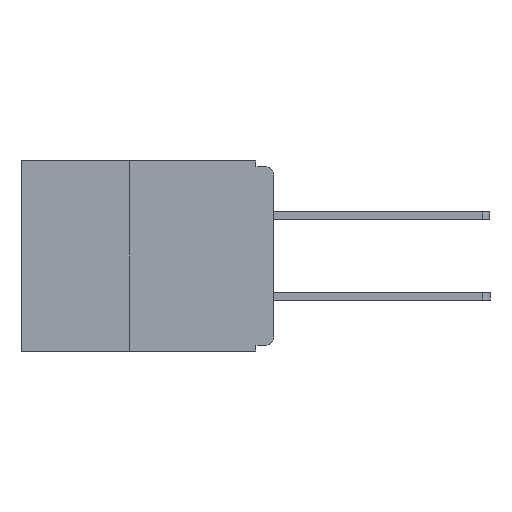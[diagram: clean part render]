
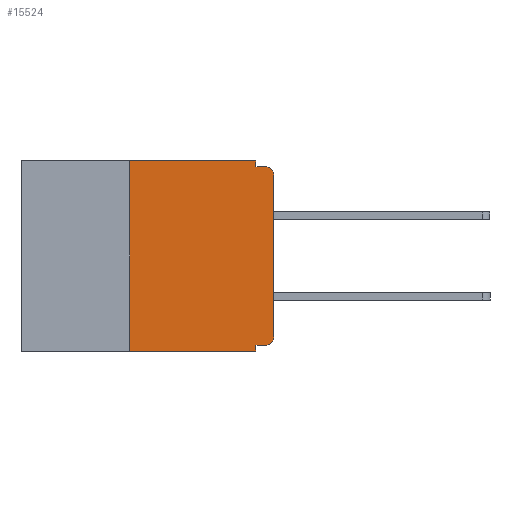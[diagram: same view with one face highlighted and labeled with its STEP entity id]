
A CAD part, left-side view. The second image highlights one B-rep face of the part: STEP entity #15524.
In plain terms, the highlighted planar face has unit normal (-1, 0, 0).
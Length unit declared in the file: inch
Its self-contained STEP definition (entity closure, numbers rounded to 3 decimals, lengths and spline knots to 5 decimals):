
#137 = EDGE_CURVE ( 'NONE', #4503, #4123, #4462, .T. ) ;
#180 = VECTOR ( 'NONE', #26298, 39.37008 ) ;
#243 = CARTESIAN_POINT ( 'NONE',  ( 0., 0.25, 0. ) ) ;
#782 = CARTESIAN_POINT ( 'NONE',  ( 0., 0.437, -0.33 ) ) ;
#796 = VERTEX_POINT ( 'NONE', #243 ) ;
#810 = ORIENTED_EDGE ( 'NONE', *, *, #29713, .T. ) ;
#937 = DIRECTION ( 'NONE',  ( 0., 1., 0. ) ) ;
#1001 = CARTESIAN_POINT ( 'NONE',  ( 0., 0.015, -0.305 ) ) ;
#1138 = EDGE_CURVE ( 'NONE', #7730, #29641, #2838, .T. ) ;
#1259 = DIRECTION ( 'NONE',  ( 0., 0., -1. ) ) ;
#1609 = LINE ( 'NONE', #21224, #26648 ) ;
#1634 = ORIENTED_EDGE ( 'NONE', *, *, #28524, .F. ) ;
#2542 = LINE ( 'NONE', #9117, #26113 ) ;
#2749 = EDGE_CURVE ( 'NONE', #7730, #796, #1609, .T. ) ;
#2838 = LINE ( 'NONE', #782, #20227 ) ;
#3063 = VERTEX_POINT ( 'NONE', #26977 ) ;
#3432 = DIRECTION ( 'NONE',  ( 0., 0., -1. ) ) ;
#3865 = LINE ( 'NONE', #23543, #8662 ) ;
#4123 = VERTEX_POINT ( 'NONE', #7746 ) ;
#4191 = DIRECTION ( 'NONE',  ( -1., 0., 0. ) ) ;
#4363 = DIRECTION ( 'NONE',  ( 0., 0., -1. ) ) ;
#4462 = LINE ( 'NONE', #20376, #23279 ) ;
#4477 = DIRECTION ( 'NONE',  ( 0., 0., -1. ) ) ;
#4503 = VERTEX_POINT ( 'NONE', #30124 ) ;
#4674 = DIRECTION ( 'NONE',  ( 0., -1., 0. ) ) ;
#5287 = ORIENTED_EDGE ( 'NONE', *, *, #26622, .T. ) ;
#6788 = CARTESIAN_POINT ( 'NONE',  ( 0., 0.25, -0.33 ) ) ;
#7091 = DIRECTION ( 'NONE',  ( 0., 0., 1. ) ) ;
#7206 = AXIS2_PLACEMENT_3D ( 'NONE', #20889, #18631, #4477 ) ;
#7514 = CARTESIAN_POINT ( 'NONE',  ( 0., 0., 0. ) ) ;
#7520 = EDGE_CURVE ( 'NONE', #19532, #4503, #20011, .T. ) ;
#7604 = FACE_OUTER_BOUND ( 'NONE', #15602, .T. ) ;
#7667 = CIRCLE ( 'NONE', #9300, 0.015 ) ;
#7730 = VERTEX_POINT ( 'NONE', #6788 ) ;
#7746 = CARTESIAN_POINT ( 'NONE',  ( 0., 0.015, -0.01 ) ) ;
#8662 = VECTOR ( 'NONE', #4674, 39.37008 ) ;
#9117 = CARTESIAN_POINT ( 'NONE',  ( 0., 0.031, -0.33 ) ) ;
#9300 = AXIS2_PLACEMENT_3D ( 'NONE', #18341, #4191, #20706 ) ;
#9545 = LINE ( 'NONE', #19789, #21333 ) ;
#10350 = EDGE_CURVE ( 'NONE', #26168, #24561, #9545, .T. ) ;
#10680 = ORIENTED_EDGE ( 'NONE', *, *, #7520, .F. ) ;
#11012 = ORIENTED_EDGE ( 'NONE', *, *, #1138, .T. ) ;
#11511 = CIRCLE ( 'NONE', #30360, 0.015 ) ;
#12250 = DIRECTION ( 'NONE',  ( 0., -1., 0. ) ) ;
#13043 = CARTESIAN_POINT ( 'NONE',  ( 0., 0.031, 0. ) ) ;
#13198 = ORIENTED_EDGE ( 'NONE', *, *, #10350, .F. ) ;
#13324 = ORIENTED_EDGE ( 'NONE', *, *, #137, .F. ) ;
#13677 = CARTESIAN_POINT ( 'NONE',  ( 0., 0., -0.305 ) ) ;
#13710 = VECTOR ( 'NONE', #1259, 39.37008 ) ;
#14464 = EDGE_CURVE ( 'NONE', #20332, #3063, #25349, .T. ) ;
#14493 = ORIENTED_EDGE ( 'NONE', *, *, #21096, .F. ) ;
#15524 = ADVANCED_FACE ( 'NONE', ( #7604 ), #27864, .F. ) ;
#15602 = EDGE_LOOP ( 'NONE', ( #30213, #810, #13324, #10680, #14493, #17505, #11012, #1634, #13198, #5287 ) ) ;
#15622 = CARTESIAN_POINT ( 'NONE',  ( 0., 0.015, -0.32 ) ) ;
#16586 = CARTESIAN_POINT ( 'NONE',  ( 0., 0.031, -0.32 ) ) ;
#17505 = ORIENTED_EDGE ( 'NONE', *, *, #2749, .F. ) ;
#17591 = DIRECTION ( 'NONE',  ( -1., 0., 0. ) ) ;
#17884 = CARTESIAN_POINT ( 'NONE',  ( 0., 0.031, 0. ) ) ;
#18341 = CARTESIAN_POINT ( 'NONE',  ( 0., 0.015, -0.025 ) ) ;
#18631 = DIRECTION ( 'NONE',  ( 1., 0., 0. ) ) ;
#19532 = VERTEX_POINT ( 'NONE', #17884 ) ;
#19789 = CARTESIAN_POINT ( 'NONE',  ( 0., 0., -0.32 ) ) ;
#20011 = LINE ( 'NONE', #13043, #13710 ) ;
#20227 = VECTOR ( 'NONE', #12250, 39.37008 ) ;
#20332 = VERTEX_POINT ( 'NONE', #13677 ) ;
#20376 = CARTESIAN_POINT ( 'NONE',  ( 0., 0., -0.01 ) ) ;
#20706 = DIRECTION ( 'NONE',  ( 0., 0., -1. ) ) ;
#20889 = CARTESIAN_POINT ( 'NONE',  ( 0., 0.437, 0. ) ) ;
#21096 = EDGE_CURVE ( 'NONE', #796, #19532, #3865, .T. ) ;
#21224 = CARTESIAN_POINT ( 'NONE',  ( 0., 0.25, -0.33 ) ) ;
#21333 = VECTOR ( 'NONE', #937, 39.37008 ) ;
#23279 = VECTOR ( 'NONE', #29741, 39.37008 ) ;
#23543 = CARTESIAN_POINT ( 'NONE',  ( 0., 0.437, 0. ) ) ;
#24561 = VERTEX_POINT ( 'NONE', #16586 ) ;
#25349 = LINE ( 'NONE', #7514, #180 ) ;
#26113 = VECTOR ( 'NONE', #4363, 39.37008 ) ;
#26168 = VERTEX_POINT ( 'NONE', #15622 ) ;
#26298 = DIRECTION ( 'NONE',  ( 0., 0., 1. ) ) ;
#26622 = EDGE_CURVE ( 'NONE', #26168, #20332, #11511, .T. ) ;
#26648 = VECTOR ( 'NONE', #7091, 39.37008 ) ;
#26977 = CARTESIAN_POINT ( 'NONE',  ( 0., 0., -0.025 ) ) ;
#27864 = PLANE ( 'NONE',  #7206 ) ;
#28524 = EDGE_CURVE ( 'NONE', #24561, #29641, #2542, .T. ) ;
#29598 = CARTESIAN_POINT ( 'NONE',  ( 0., 0.031, -0.33 ) ) ;
#29641 = VERTEX_POINT ( 'NONE', #29598 ) ;
#29713 = EDGE_CURVE ( 'NONE', #3063, #4123, #7667, .T. ) ;
#29741 = DIRECTION ( 'NONE',  ( 0., -1., 0. ) ) ;
#30124 = CARTESIAN_POINT ( 'NONE',  ( 0., 0.031, -0.01 ) ) ;
#30213 = ORIENTED_EDGE ( 'NONE', *, *, #14464, .T. ) ;
#30360 = AXIS2_PLACEMENT_3D ( 'NONE', #1001, #17591, #3432 ) ;
